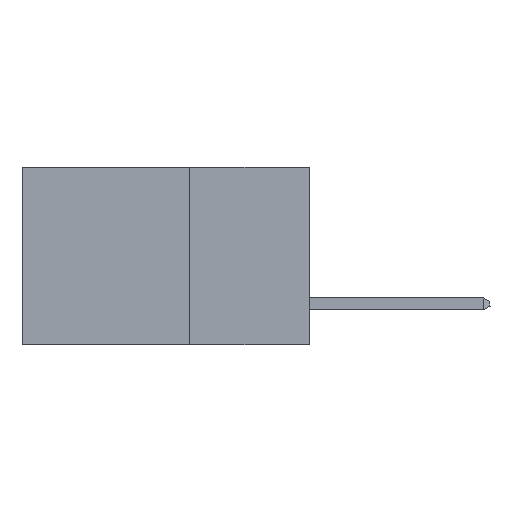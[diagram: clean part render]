
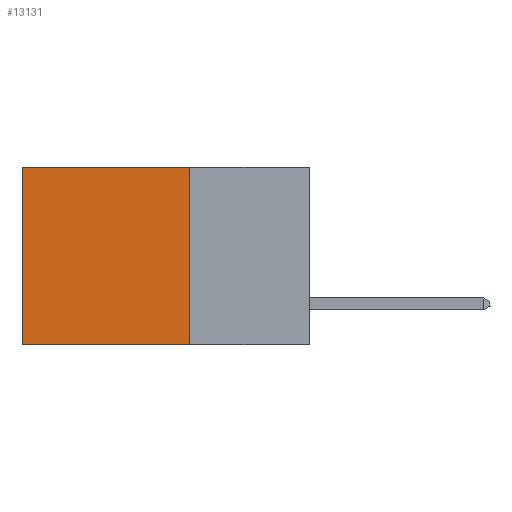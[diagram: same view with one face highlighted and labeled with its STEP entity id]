
A CAD part, left-side view. The second image highlights one B-rep face of the part: STEP entity #13131.
In plain terms, the highlighted planar face has unit normal (-1, 0, 0).
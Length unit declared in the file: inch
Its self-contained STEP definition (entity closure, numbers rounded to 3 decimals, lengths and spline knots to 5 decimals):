
#703 = VERTEX_POINT ( 'NONE', #6240 ) ;
#1502 = CARTESIAN_POINT ( 'NONE',  ( 0.2875, 0.25, -0.37 ) ) ;
#2540 = CARTESIAN_POINT ( 'NONE',  ( 0.2875, 0.25, 0. ) ) ;
#2641 = LINE ( 'NONE', #7553, #17812 ) ;
#2663 = ORIENTED_EDGE ( 'NONE', *, *, #11209, .T. ) ;
#3008 = VERTEX_POINT ( 'NONE', #1502 ) ;
#3336 = DIRECTION ( 'NONE',  ( 1., 0., 0. ) ) ;
#3447 = LINE ( 'NONE', #12127, #6313 ) ;
#4065 = EDGE_CURVE ( 'NONE', #3008, #703, #2641, .T. ) ;
#4803 = ORIENTED_EDGE ( 'NONE', *, *, #5458, .T. ) ;
#5246 = CARTESIAN_POINT ( 'NONE',  ( 0.2875, 0.6, 0. ) ) ;
#5458 = EDGE_CURVE ( 'NONE', #19106, #703, #15674, .T. ) ;
#5708 = VECTOR ( 'NONE', #7608, 39.37008 ) ;
#6240 = CARTESIAN_POINT ( 'NONE',  ( 0.2875, 0.6, -0.37 ) ) ;
#6313 = VECTOR ( 'NONE', #18962, 39.37008 ) ;
#6567 = AXIS2_PLACEMENT_3D ( 'NONE', #13342, #3336, #8076 ) ;
#7553 = CARTESIAN_POINT ( 'NONE',  ( 0.2875, 0.25, -0.37 ) ) ;
#7568 = EDGE_LOOP ( 'NONE', ( #4803, #10590, #11332, #2663 ) ) ;
#7608 = DIRECTION ( 'NONE',  ( 0., 0., -1. ) ) ;
#7749 = FACE_OUTER_BOUND ( 'NONE', #7568, .T. ) ;
#8076 = DIRECTION ( 'NONE',  ( 0., 0., -1. ) ) ;
#10031 = CARTESIAN_POINT ( 'NONE',  ( 0.2875, 0.25, 0. ) ) ;
#10590 = ORIENTED_EDGE ( 'NONE', *, *, #4065, .F. ) ;
#11209 = EDGE_CURVE ( 'NONE', #17565, #19106, #11727, .T. ) ;
#11332 = ORIENTED_EDGE ( 'NONE', *, *, #18561, .F. ) ;
#11557 = DIRECTION ( 'NONE',  ( 0., 1., 0. ) ) ;
#11727 = LINE ( 'NONE', #10031, #19888 ) ;
#11729 = PLANE ( 'NONE',  #6567 ) ;
#12127 = CARTESIAN_POINT ( 'NONE',  ( 0.2875, 0.25, 0. ) ) ;
#13131 = ADVANCED_FACE ( 'NONE', ( #7749 ), #11729, .F. ) ;
#13342 = CARTESIAN_POINT ( 'NONE',  ( 0.2875, 0.25, 0. ) ) ;
#15674 = LINE ( 'NONE', #20956, #5708 ) ;
#17565 = VERTEX_POINT ( 'NONE', #2540 ) ;
#17656 = DIRECTION ( 'NONE',  ( 0., 1., 0. ) ) ;
#17812 = VECTOR ( 'NONE', #17656, 39.37008 ) ;
#18561 = EDGE_CURVE ( 'NONE', #17565, #3008, #3447, .T. ) ;
#18962 = DIRECTION ( 'NONE',  ( 0., 0., -1. ) ) ;
#19106 = VERTEX_POINT ( 'NONE', #5246 ) ;
#19888 = VECTOR ( 'NONE', #11557, 39.37008 ) ;
#20956 = CARTESIAN_POINT ( 'NONE',  ( 0.2875, 0.6, 0. ) ) ;
